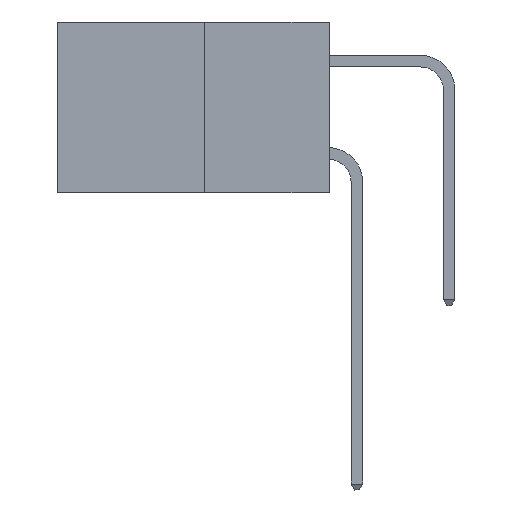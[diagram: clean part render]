
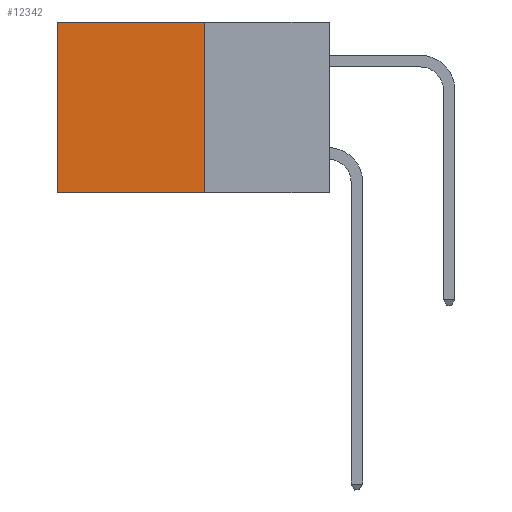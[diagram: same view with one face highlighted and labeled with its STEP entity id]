
A CAD part, left-side view. The second image highlights one B-rep face of the part: STEP entity #12342.
In plain terms, the highlighted planar face has unit normal (-1, 0, 0).
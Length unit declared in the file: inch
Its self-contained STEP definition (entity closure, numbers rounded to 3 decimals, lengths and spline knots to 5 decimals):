
#1001 = VERTEX_POINT ( 'NONE', #7750 ) ;
#1499 = FACE_OUTER_BOUND ( 'NONE', #9827, .T. ) ;
#1952 = DIRECTION ( 'NONE',  ( 0., 0., -1. ) ) ;
#2021 = EDGE_CURVE ( 'NONE', #4496, #1001, #6604, .T. ) ;
#2201 = VERTEX_POINT ( 'NONE', #10112 ) ;
#2525 = VECTOR ( 'NONE', #11845, 39.37008 ) ;
#3193 = LINE ( 'NONE', #4910, #9334 ) ;
#3434 = ORIENTED_EDGE ( 'NONE', *, *, #12670, .T. ) ;
#4496 = VERTEX_POINT ( 'NONE', #13225 ) ;
#4826 = DIRECTION ( 'NONE',  ( 0., 0., -1. ) ) ;
#4910 = CARTESIAN_POINT ( 'NONE',  ( 0.277, 0.27, -0.37 ) ) ;
#4930 = EDGE_CURVE ( 'NONE', #2201, #1001, #8357, .T. ) ;
#5038 = EDGE_CURVE ( 'NONE', #8581, #4496, #3193, .T. ) ;
#6421 = DIRECTION ( 'NONE',  ( 0., 0., -1. ) ) ;
#6464 = ORIENTED_EDGE ( 'NONE', *, *, #4930, .T. ) ;
#6526 = CARTESIAN_POINT ( 'NONE',  ( 0.277, 0.59, -0.37 ) ) ;
#6604 = LINE ( 'NONE', #12704, #2525 ) ;
#6800 = VECTOR ( 'NONE', #13460, 39.37008 ) ;
#7750 = CARTESIAN_POINT ( 'NONE',  ( 0.277, 0.59, -0.37 ) ) ;
#7908 = CARTESIAN_POINT ( 'NONE',  ( 0.277, 0.27, 0. ) ) ;
#8161 = CARTESIAN_POINT ( 'NONE',  ( 0.277, 0.27, -0.37 ) ) ;
#8357 = LINE ( 'NONE', #6526, #13839 ) ;
#8581 = VERTEX_POINT ( 'NONE', #7908 ) ;
#9293 = ORIENTED_EDGE ( 'NONE', *, *, #5038, .F. ) ;
#9334 = VECTOR ( 'NONE', #4826, 39.37008 ) ;
#9445 = DIRECTION ( 'NONE',  ( 1., 0., 0. ) ) ;
#9827 = EDGE_LOOP ( 'NONE', ( #6464, #10702, #9293, #3434 ) ) ;
#10112 = CARTESIAN_POINT ( 'NONE',  ( 0.277, 0.59, 0. ) ) ;
#10702 = ORIENTED_EDGE ( 'NONE', *, *, #2021, .F. ) ;
#11845 = DIRECTION ( 'NONE',  ( 0., 1., 0. ) ) ;
#12288 = CARTESIAN_POINT ( 'NONE',  ( 0.277, 0.27, 0. ) ) ;
#12342 = ADVANCED_FACE ( 'NONE', ( #1499 ), #15169, .F. ) ;
#12670 = EDGE_CURVE ( 'NONE', #8581, #2201, #13156, .T. ) ;
#12704 = CARTESIAN_POINT ( 'NONE',  ( 0.277, 0.27, -0.37 ) ) ;
#13156 = LINE ( 'NONE', #12288, #6800 ) ;
#13225 = CARTESIAN_POINT ( 'NONE',  ( 0.277, 0.27, -0.37 ) ) ;
#13460 = DIRECTION ( 'NONE',  ( 0., 1., 0. ) ) ;
#13538 = AXIS2_PLACEMENT_3D ( 'NONE', #8161, #9445, #1952 ) ;
#13839 = VECTOR ( 'NONE', #6421, 39.37008 ) ;
#15169 = PLANE ( 'NONE',  #13538 ) ;
